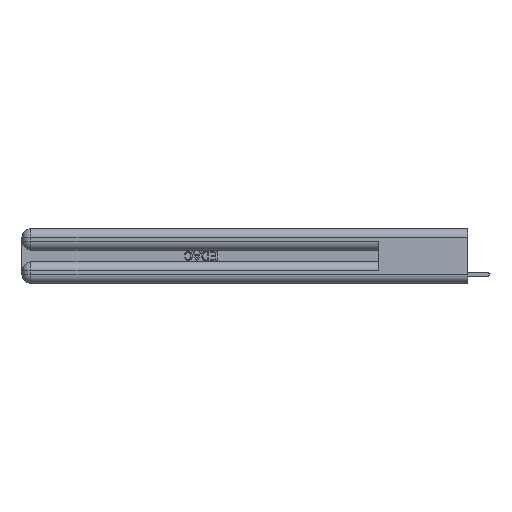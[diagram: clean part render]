
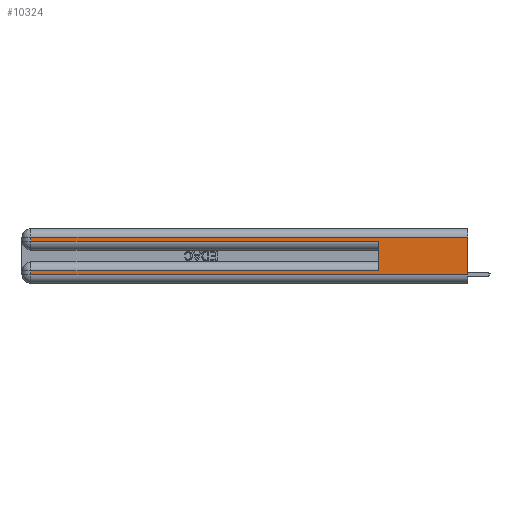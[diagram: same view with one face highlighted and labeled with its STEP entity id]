
A CAD part, left-side view. The second image highlights one B-rep face of the part: STEP entity #10324.
In plain terms, the highlighted planar face has unit normal (-1, 0, 0).
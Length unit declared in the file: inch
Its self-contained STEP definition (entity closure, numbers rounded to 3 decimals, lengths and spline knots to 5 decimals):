
#753 = LINE ( 'NONE', #30393, #6524 ) ;
#998 = EDGE_CURVE ( 'NONE', #7245, #26487, #13943, .T. ) ;
#1665 = ORIENTED_EDGE ( 'NONE', *, *, #22016, .T. ) ;
#1895 = LINE ( 'NONE', #13771, #31641 ) ;
#1908 = CARTESIAN_POINT ( 'NONE',  ( 0., 0., 0.085 ) ) ;
#2157 = EDGE_CURVE ( 'NONE', #7245, #20838, #34095, .T. ) ;
#2263 = EDGE_CURVE ( 'NONE', #29544, #26487, #13011, .T. ) ;
#3001 = CARTESIAN_POINT ( 'NONE',  ( 0., 2.94, 0.37 ) ) ;
#3709 = DIRECTION ( 'NONE',  ( 0., 1., 0. ) ) ;
#6098 = DIRECTION ( 'NONE',  ( 0., 0., 1. ) ) ;
#6524 = VECTOR ( 'NONE', #22578, 39.37008 ) ;
#7245 = VERTEX_POINT ( 'NONE', #14303 ) ;
#7902 = PLANE ( 'NONE',  #30314 ) ;
#7970 = CARTESIAN_POINT ( 'NONE',  ( 0., 2.94, 0.31 ) ) ;
#8150 = ORIENTED_EDGE ( 'NONE', *, *, #2157, .T. ) ;
#8326 = VERTEX_POINT ( 'NONE', #13953 ) ;
#8560 = LINE ( 'NONE', #1908, #24301 ) ;
#9013 = EDGE_CURVE ( 'NONE', #9541, #32115, #753, .T. ) ;
#9119 = ORIENTED_EDGE ( 'NONE', *, *, #9013, .T. ) ;
#9541 = VERTEX_POINT ( 'NONE', #31538 ) ;
#9919 = CARTESIAN_POINT ( 'NONE',  ( 0., 2.94, 0.085 ) ) ;
#10324 = ADVANCED_FACE ( 'NONE', ( #12863 ), #7902, .F. ) ;
#10589 = CARTESIAN_POINT ( 'NONE',  ( 0., 0., 0.06 ) ) ;
#12863 = FACE_OUTER_BOUND ( 'NONE', #27117, .T. ) ;
#13011 = LINE ( 'NONE', #10589, #29549 ) ;
#13394 = CARTESIAN_POINT ( 'NONE',  ( 0., 0., 0.06 ) ) ;
#13657 = LINE ( 'NONE', #13871, #26024 ) ;
#13771 = CARTESIAN_POINT ( 'NONE',  ( 0., 2.94, 0.37 ) ) ;
#13871 = CARTESIAN_POINT ( 'NONE',  ( 0., 0.6, 0.145 ) ) ;
#13943 = LINE ( 'NONE', #28536, #33344 ) ;
#13953 = CARTESIAN_POINT ( 'NONE',  ( 0., 0.6, 0.085 ) ) ;
#14303 = CARTESIAN_POINT ( 'NONE',  ( 0., 0., 0.31 ) ) ;
#15151 = ORIENTED_EDGE ( 'NONE', *, *, #33610, .T. ) ;
#15183 = DIRECTION ( 'NONE',  ( 0., 1., 0. ) ) ;
#16402 = DIRECTION ( 'NONE',  ( 0., 0., -1. ) ) ;
#16512 = VECTOR ( 'NONE', #29773, 39.37008 ) ;
#18844 = ORIENTED_EDGE ( 'NONE', *, *, #25820, .T. ) ;
#19538 = CARTESIAN_POINT ( 'NONE',  ( 0., 0., 0.31 ) ) ;
#20838 = VERTEX_POINT ( 'NONE', #7970 ) ;
#22016 = EDGE_CURVE ( 'NONE', #24298, #29544, #24386, .T. ) ;
#22578 = DIRECTION ( 'NONE',  ( 0., -1., 0. ) ) ;
#23569 = CARTESIAN_POINT ( 'NONE',  ( 0., 0.6, 0.285 ) ) ;
#24034 = ORIENTED_EDGE ( 'NONE', *, *, #29425, .F. ) ;
#24298 = VERTEX_POINT ( 'NONE', #9919 ) ;
#24301 = VECTOR ( 'NONE', #15183, 39.37008 ) ;
#24386 = LINE ( 'NONE', #3001, #16512 ) ;
#24821 = CARTESIAN_POINT ( 'NONE',  ( 0., 2.94, 0.06 ) ) ;
#25820 = EDGE_CURVE ( 'NONE', #8326, #24298, #8560, .T. ) ;
#26024 = VECTOR ( 'NONE', #6098, 39.37008 ) ;
#26242 = CARTESIAN_POINT ( 'NONE',  ( 0., 0., 0.37 ) ) ;
#26349 = DIRECTION ( 'NONE',  ( 1., 0., 0. ) ) ;
#26487 = VERTEX_POINT ( 'NONE', #13394 ) ;
#27091 = VECTOR ( 'NONE', #3709, 39.37008 ) ;
#27117 = EDGE_LOOP ( 'NONE', ( #32823, #8150, #15151, #9119, #24034, #18844, #1665, #31004 ) ) ;
#28420 = DIRECTION ( 'NONE',  ( 0., 0., -1. ) ) ;
#28536 = CARTESIAN_POINT ( 'NONE',  ( 0., 0., 0.37 ) ) ;
#29425 = EDGE_CURVE ( 'NONE', #8326, #32115, #13657, .T. ) ;
#29544 = VERTEX_POINT ( 'NONE', #24821 ) ;
#29549 = VECTOR ( 'NONE', #31523, 39.37008 ) ;
#29773 = DIRECTION ( 'NONE',  ( 0., 0., -1. ) ) ;
#30314 = AXIS2_PLACEMENT_3D ( 'NONE', #26242, #26349, #31220 ) ;
#30393 = CARTESIAN_POINT ( 'NONE',  ( 0., 0., 0.285 ) ) ;
#31004 = ORIENTED_EDGE ( 'NONE', *, *, #2263, .T. ) ;
#31220 = DIRECTION ( 'NONE',  ( 0., 0., -1. ) ) ;
#31523 = DIRECTION ( 'NONE',  ( 0., -1., 0. ) ) ;
#31538 = CARTESIAN_POINT ( 'NONE',  ( 0., 2.94, 0.285 ) ) ;
#31641 = VECTOR ( 'NONE', #16402, 39.37008 ) ;
#32115 = VERTEX_POINT ( 'NONE', #23569 ) ;
#32823 = ORIENTED_EDGE ( 'NONE', *, *, #998, .F. ) ;
#33344 = VECTOR ( 'NONE', #28420, 39.37008 ) ;
#33610 = EDGE_CURVE ( 'NONE', #20838, #9541, #1895, .T. ) ;
#34095 = LINE ( 'NONE', #19538, #27091 ) ;
